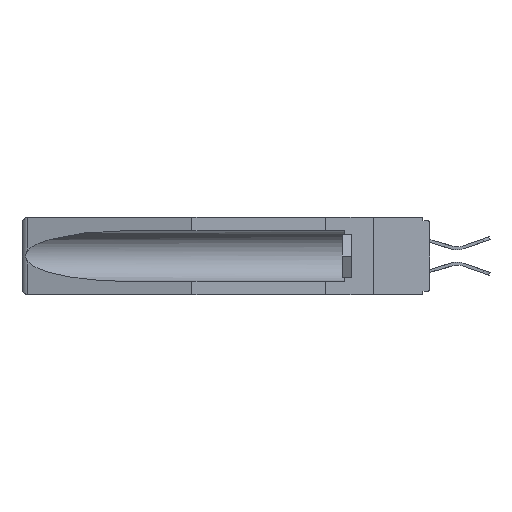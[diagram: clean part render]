
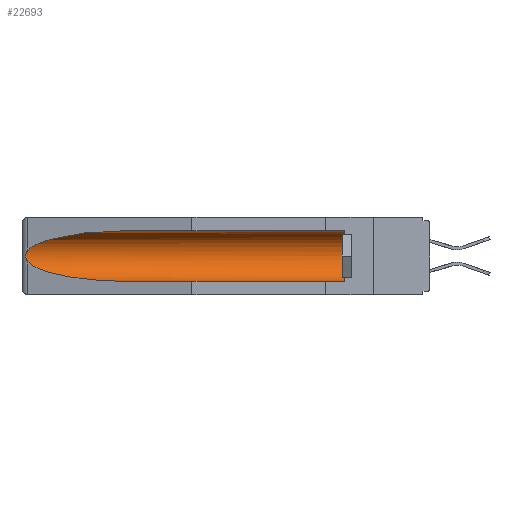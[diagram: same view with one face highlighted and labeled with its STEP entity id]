
A CAD part, left-side view. The second image highlights one B-rep face of the part: STEP entity #22693.
In plain terms, the highlighted cylindrical face has radius 2.857 mm (diameter 5.715 mm), a partial arc.
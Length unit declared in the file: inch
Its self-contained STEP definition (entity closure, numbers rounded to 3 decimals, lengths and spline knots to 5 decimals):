
#249 = CARTESIAN_POINT ( 'NONE',  ( 0.26597, 1.52961, -0.15275 ) ) ;
#415 = CARTESIAN_POINT ( 'NONE',  ( 0.2675, 1.53308, -0.16763 ) ) ;
#816 = CARTESIAN_POINT ( 'NONE',  ( 0.155, 1.07973, -0.284 ) ) ;
#1239 = VERTEX_POINT ( 'NONE', #8042 ) ;
#1427 = ORIENTED_EDGE ( 'NONE', *, *, #26045, .T. ) ;
#2528 = CYLINDRICAL_SURFACE ( 'NONE', #12675, 0.1125 ) ;
#2632 = ORIENTED_EDGE ( 'NONE', *, *, #15187, .F. ) ;
#3607 = AXIS2_PLACEMENT_3D ( 'NONE', #5629, #22632, #9912 ) ;
#3782 = CARTESIAN_POINT ( 'NONE',  ( 0.155, 1.07973, -0.284 ) ) ;
#4600 = CARTESIAN_POINT ( 'NONE',  ( 0.26597, 1.5296, -0.19026 ) ) ;
#5014 = CARTESIAN_POINT ( 'NONE',  ( 0.25451, 1.48313, -0.09465 ) ) ;
#5195 = CARTESIAN_POINT ( 'NONE',  ( 0.21114, 1.30732, -0.059 ) ) ;
#5629 = CARTESIAN_POINT ( 'NONE',  ( 0.155, 0.126, -0.1715 ) ) ;
#6654 = CARTESIAN_POINT ( 'NONE',  ( 0.2673, 1.5327, -0.16383 ) ) ;
#7160 = CARTESIAN_POINT ( 'NONE',  ( 0.21114, 1.30732, -0.284 ) ) ;
#7415 = LINE ( 'NONE', #15364, #18732 ) ;
#8042 = CARTESIAN_POINT ( 'NONE',  ( 0.26537, 1.52718, -0.19328 ) ) ;
#8861 = CARTESIAN_POINT ( 'NONE',  ( 0.26655, 1.53094, -0.18657 ) ) ;
#8865 =( BOUNDED_CURVE ( )  B_SPLINE_CURVE ( 3, ( #17119, #21395, #7160, #816 ),
 .UNSPECIFIED., .F., .F. ) 
 B_SPLINE_CURVE_WITH_KNOTS ( ( 4, 4 ),
 ( 0.1948, 1.5708 ),
 .UNSPECIFIED. ) 
 CURVE ( )  GEOMETRIC_REPRESENTATION_ITEM ( )  RATIONAL_B_SPLINE_CURVE ( ( 1., 0.848, 0.848, 1. ) ) 
 REPRESENTATION_ITEM ( '' )  );
#9882 = EDGE_CURVE ( 'NONE', #22192, #10963, #15186, .T. ) ;
#9912 = DIRECTION ( 'NONE',  ( 0., 0., 1. ) ) ;
#10800 = VECTOR ( 'NONE', #15072, 39.37008 ) ;
#10963 = VERTEX_POINT ( 'NONE', #24120 ) ;
#11510 = CARTESIAN_POINT ( 'NONE',  ( 0.26537, 1.52718, -0.14972 ) ) ;
#11810 = EDGE_CURVE ( 'NONE', #16992, #1239, #26221, .T. ) ;
#12530 = ORIENTED_EDGE ( 'NONE', *, *, #16448, .T. ) ;
#12675 = AXIS2_PLACEMENT_3D ( 'NONE', #25497, #21140, #19002 ) ;
#12756 = CARTESIAN_POINT ( 'NONE',  ( 0.26654, 1.53092, -0.15636 ) ) ;
#12824 = CARTESIAN_POINT ( 'NONE',  ( 0.155, 1.07973, -0.059 ) ) ;
#13419 = CARTESIAN_POINT ( 'NONE',  ( 0.26537, 1.52718, -0.14972 ) ) ;
#14122 = VERTEX_POINT ( 'NONE', #12824 ) ;
#15005 = DIRECTION ( 'NONE',  ( 0., 1., 0. ) ) ;
#15072 = DIRECTION ( 'NONE',  ( 0., 1., 0. ) ) ;
#15186 = CIRCLE ( 'NONE', #3607, 0.1125 ) ;
#15187 = EDGE_CURVE ( 'NONE', #22192, #18567, #15785, .T. ) ;
#15364 = CARTESIAN_POINT ( 'NONE',  ( 0.155, -0.30754, -0.059 ) ) ;
#15785 = LINE ( 'NONE', #25760, #10800 ) ;
#16448 = EDGE_CURVE ( 'NONE', #10963, #14122, #7415, .T. ) ;
#16992 = VERTEX_POINT ( 'NONE', #13419 ) ;
#17079 = CARTESIAN_POINT ( 'NONE',  ( 0.155, 0.126, -0.284 ) ) ;
#17119 = CARTESIAN_POINT ( 'NONE',  ( 0.26537, 1.52718, -0.19328 ) ) ;
#17137 = CARTESIAN_POINT ( 'NONE',  ( 0.26537, 1.52718, -0.19328 ) ) ;
#17412 = CARTESIAN_POINT ( 'NONE',  ( 0.26537, 1.52718, -0.14972 ) ) ;
#18567 = VERTEX_POINT ( 'NONE', #3782 ) ;
#18732 = VECTOR ( 'NONE', #15005, 39.37008 ) ;
#19002 = DIRECTION ( 'NONE',  ( 0., 0., 1. ) ) ;
#19194 = ORIENTED_EDGE ( 'NONE', *, *, #11810, .T. ) ;
#19692 = EDGE_CURVE ( 'NONE', #1239, #18567, #8865, .T. ) ;
#21140 = DIRECTION ( 'NONE',  ( 0., 1., 0. ) ) ;
#21376 = ORIENTED_EDGE ( 'NONE', *, *, #19692, .T. ) ;
#21395 = CARTESIAN_POINT ( 'NONE',  ( 0.25451, 1.48313, -0.24835 ) ) ;
#21586 = CARTESIAN_POINT ( 'NONE',  ( 0.2673, 1.53269, -0.17917 ) ) ;
#21671 = CARTESIAN_POINT ( 'NONE',  ( 0.2675, 1.53308, -0.17534 ) ) ;
#22192 = VERTEX_POINT ( 'NONE', #17079 ) ;
#22632 = DIRECTION ( 'NONE',  ( 0., -1., 0. ) ) ;
#22693 = ADVANCED_FACE ( 'NONE', ( #23074 ), #2528, .F. ) ;
#23074 = FACE_OUTER_BOUND ( 'NONE', #23274, .T. ) ;
#23274 = EDGE_LOOP ( 'NONE', ( #1427, #19194, #21376, #2632, #24432, #12530 ) ) ;
#24120 = CARTESIAN_POINT ( 'NONE',  ( 0.155, 0.126, -0.059 ) ) ;
#24432 = ORIENTED_EDGE ( 'NONE', *, *, #9882, .T. ) ;
#25497 = CARTESIAN_POINT ( 'NONE',  ( 0.155, -0.30754, -0.1715 ) ) ;
#25760 = CARTESIAN_POINT ( 'NONE',  ( 0.155, -0.30754, -0.284 ) ) ;
#26045 = EDGE_CURVE ( 'NONE', #14122, #16992, #27050, .T. ) ;
#26221 = B_SPLINE_CURVE_WITH_KNOTS ( 'NONE', 3,
 ( #17412, #249, #12756, #6654, #415, #21671, #21586, #8861, #4600, #17137 ),
 .UNSPECIFIED., .F., .F.,
 ( 4, 2, 2, 2, 4 ),
 ( 0., 0.00029, 0.00058, 0.00087, 0.00117 ),
 .UNSPECIFIED. ) ;
#26460 = CARTESIAN_POINT ( 'NONE',  ( 0.155, 1.07973, -0.059 ) ) ;
#27050 =( BOUNDED_CURVE ( )  B_SPLINE_CURVE ( 3, ( #26460, #5195, #5014, #11510 ),
 .UNSPECIFIED., .F., .F. ) 
 B_SPLINE_CURVE_WITH_KNOTS ( ( 4, 4 ),
 ( 4.71239, 6.08839 ),
 .UNSPECIFIED. ) 
 CURVE ( )  GEOMETRIC_REPRESENTATION_ITEM ( )  RATIONAL_B_SPLINE_CURVE ( ( 1., 0.848, 0.848, 1. ) ) 
 REPRESENTATION_ITEM ( '' )  );
